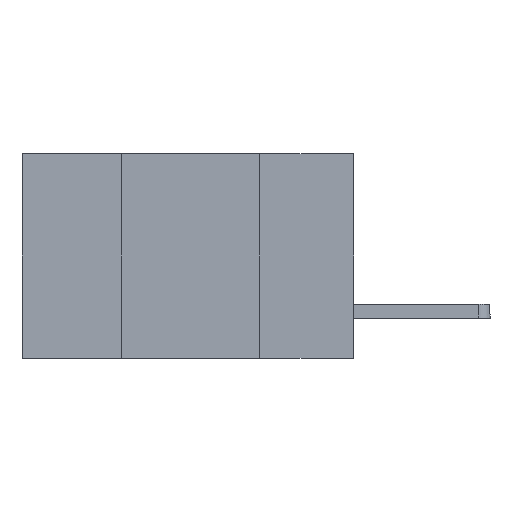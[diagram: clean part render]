
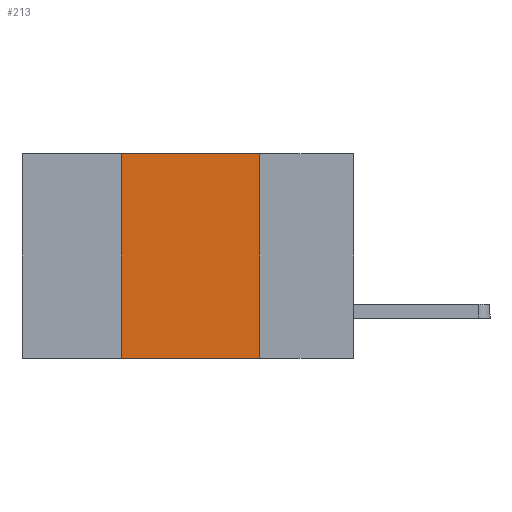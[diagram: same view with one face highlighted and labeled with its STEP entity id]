
A CAD part, left-side view. The second image highlights one B-rep face of the part: STEP entity #213.
In plain terms, the highlighted planar face has unit normal (-1, 0, 0).
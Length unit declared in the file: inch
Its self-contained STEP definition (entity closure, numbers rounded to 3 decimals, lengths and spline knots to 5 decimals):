
#11 = FACE_OUTER_BOUND ( 'NONE', #5615, .T. ) ;
#176 = VECTOR ( 'NONE', #5743, 39.37008 ) ;
#213 = ADVANCED_FACE ( 'NONE', ( #11 ), #7430, .F. ) ;
#460 = EDGE_CURVE ( 'NONE', #6345, #4170, #9396, .T. ) ;
#651 = DIRECTION ( 'NONE',  ( 0., 0., 1. ) ) ;
#956 = VERTEX_POINT ( 'NONE', #1573 ) ;
#1061 = LINE ( 'NONE', #11001, #5675 ) ;
#1573 = CARTESIAN_POINT ( 'NONE',  ( 0., 0.42, 0. ) ) ;
#3925 = CARTESIAN_POINT ( 'NONE',  ( 0., 0.42, -0.37 ) ) ;
#4012 = EDGE_CURVE ( 'NONE', #4210, #4170, #8854, .T. ) ;
#4170 = VERTEX_POINT ( 'NONE', #4617 ) ;
#4200 = CARTESIAN_POINT ( 'NONE',  ( 0., 0.17, 0. ) ) ;
#4210 = VERTEX_POINT ( 'NONE', #3925 ) ;
#4533 = VECTOR ( 'NONE', #9904, 39.37008 ) ;
#4617 = CARTESIAN_POINT ( 'NONE',  ( 0., 0.17, -0.37 ) ) ;
#5556 = CARTESIAN_POINT ( 'NONE',  ( 0., 0.17, 0. ) ) ;
#5615 = EDGE_LOOP ( 'NONE', ( #8839, #10367, #10148, #7389 ) ) ;
#5675 = VECTOR ( 'NONE', #651, 39.37008 ) ;
#5743 = DIRECTION ( 'NONE',  ( 0., 0., -1. ) ) ;
#6345 = VERTEX_POINT ( 'NONE', #4200 ) ;
#6978 = DIRECTION ( 'NONE',  ( 0., -1., 0. ) ) ;
#6990 = CARTESIAN_POINT ( 'NONE',  ( 0., 0.6, -0.37 ) ) ;
#7338 = DIRECTION ( 'NONE',  ( 0., 0., -1. ) ) ;
#7351 = DIRECTION ( 'NONE',  ( 1., 0., 0. ) ) ;
#7383 = CARTESIAN_POINT ( 'NONE',  ( 0., 0.6, 0. ) ) ;
#7389 = ORIENTED_EDGE ( 'NONE', *, *, #4012, .T. ) ;
#7430 = PLANE ( 'NONE',  #8791 ) ;
#7470 = CARTESIAN_POINT ( 'NONE',  ( 0., 0.6, 0. ) ) ;
#8791 = AXIS2_PLACEMENT_3D ( 'NONE', #7470, #7351, #7338 ) ;
#8839 = ORIENTED_EDGE ( 'NONE', *, *, #460, .F. ) ;
#8854 = LINE ( 'NONE', #6990, #10873 ) ;
#9186 = LINE ( 'NONE', #7383, #4533 ) ;
#9396 = LINE ( 'NONE', #5556, #176 ) ;
#9904 = DIRECTION ( 'NONE',  ( 0., -1., 0. ) ) ;
#10111 = EDGE_CURVE ( 'NONE', #956, #6345, #9186, .T. ) ;
#10148 = ORIENTED_EDGE ( 'NONE', *, *, #10434, .F. ) ;
#10367 = ORIENTED_EDGE ( 'NONE', *, *, #10111, .F. ) ;
#10434 = EDGE_CURVE ( 'NONE', #4210, #956, #1061, .T. ) ;
#10873 = VECTOR ( 'NONE', #6978, 39.37008 ) ;
#11001 = CARTESIAN_POINT ( 'NONE',  ( 0., 0.42, 0. ) ) ;
